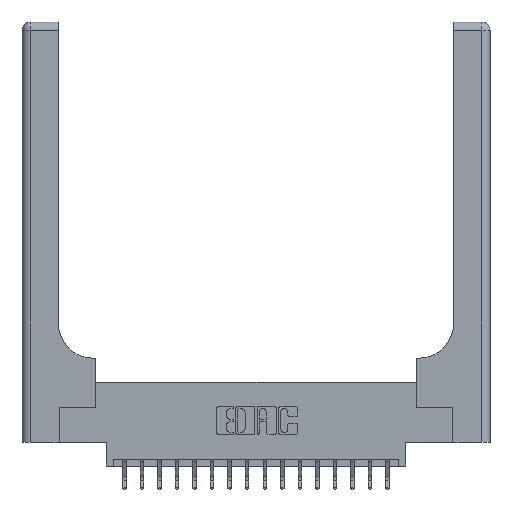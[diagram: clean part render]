
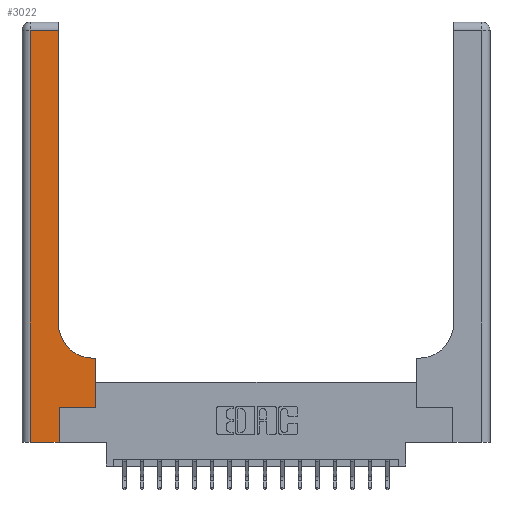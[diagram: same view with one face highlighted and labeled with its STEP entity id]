
A CAD part, top view. The second image highlights one B-rep face of the part: STEP entity #3022.
In plain terms, the highlighted planar face has unit normal (0, 0, 1).
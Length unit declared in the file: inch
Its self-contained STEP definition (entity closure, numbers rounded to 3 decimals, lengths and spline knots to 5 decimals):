
#124 = VECTOR ( 'NONE', #13256, 39.37008 ) ;
#356 = AXIS2_PLACEMENT_3D ( 'NONE', #17560, #8600, #19042 ) ;
#387 = CIRCLE ( 'NONE', #356, 0.25 ) ;
#470 = CARTESIAN_POINT ( 'NONE',  ( 0.26, 2.94, 0.37 ) ) ;
#877 = DIRECTION ( 'NONE',  ( -1., 0., 0. ) ) ;
#941 = EDGE_LOOP ( 'NONE', ( #1233, #9924, #9401, #5810, #12615, #2392, #7498, #4739, #6015 ) ) ;
#948 = CARTESIAN_POINT ( 'NONE',  ( 0.265, 0.25, 0.37 ) ) ;
#1233 = ORIENTED_EDGE ( 'NONE', *, *, #8392, .T. ) ;
#1277 = VERTEX_POINT ( 'NONE', #470 ) ;
#1397 = CARTESIAN_POINT ( 'NONE',  ( 0.06, 2.94, 0.37 ) ) ;
#1507 = CARTESIAN_POINT ( 'NONE',  ( 0.26, 0.85, 0.37 ) ) ;
#1747 = EDGE_CURVE ( 'NONE', #13951, #7354, #18342, .T. ) ;
#1796 = DIRECTION ( 'NONE',  ( 0., 1., 0. ) ) ;
#2098 = VERTEX_POINT ( 'NONE', #19387 ) ;
#2392 = ORIENTED_EDGE ( 'NONE', *, *, #11087, .T. ) ;
#2515 = CARTESIAN_POINT ( 'NONE',  ( 0.26, 0.6, 0.37 ) ) ;
#2745 = CARTESIAN_POINT ( 'NONE',  ( 0.06, 3., 0.37 ) ) ;
#3022 = ADVANCED_FACE ( 'NONE', ( #7053 ), #17415, .F. ) ;
#3240 = VERTEX_POINT ( 'NONE', #1397 ) ;
#3827 = LINE ( 'NONE', #2515, #18836 ) ;
#4114 = VECTOR ( 'NONE', #15551, 39.37008 ) ;
#4638 = CARTESIAN_POINT ( 'NONE',  ( 0.51, 0.6, 0.37 ) ) ;
#4739 = ORIENTED_EDGE ( 'NONE', *, *, #7251, .T. ) ;
#5372 = EDGE_CURVE ( 'NONE', #11642, #6927, #10032, .T. ) ;
#5810 = ORIENTED_EDGE ( 'NONE', *, *, #16534, .T. ) ;
#6015 = ORIENTED_EDGE ( 'NONE', *, *, #15964, .T. ) ;
#6381 = VECTOR ( 'NONE', #1796, 39.37008 ) ;
#6927 = VERTEX_POINT ( 'NONE', #9258 ) ;
#7053 = FACE_OUTER_BOUND ( 'NONE', #941, .T. ) ;
#7251 = EDGE_CURVE ( 'NONE', #6927, #12770, #3827, .T. ) ;
#7315 = LINE ( 'NONE', #948, #17858 ) ;
#7354 = VERTEX_POINT ( 'NONE', #17809 ) ;
#7498 = ORIENTED_EDGE ( 'NONE', *, *, #5372, .T. ) ;
#8170 = CARTESIAN_POINT ( 'NONE',  ( 0.265, 0., 0.37 ) ) ;
#8392 = EDGE_CURVE ( 'NONE', #18990, #1277, #12119, .T. ) ;
#8447 = CARTESIAN_POINT ( 'NONE',  ( 0., 3., 0.37 ) ) ;
#8600 = DIRECTION ( 'NONE',  ( 0., 0., -1. ) ) ;
#9258 = CARTESIAN_POINT ( 'NONE',  ( 0.528, 0.6, 0.37 ) ) ;
#9401 = ORIENTED_EDGE ( 'NONE', *, *, #11819, .T. ) ;
#9924 = ORIENTED_EDGE ( 'NONE', *, *, #13199, .T. ) ;
#9960 = DIRECTION ( 'NONE',  ( 0., 0., -1. ) ) ;
#10032 = LINE ( 'NONE', #14235, #10484 ) ;
#10038 = DIRECTION ( 'NONE',  ( -1., 0., 0. ) ) ;
#10258 = DIRECTION ( 'NONE',  ( 0., -1., 0. ) ) ;
#10350 = VECTOR ( 'NONE', #14552, 39.37008 ) ;
#10484 = VECTOR ( 'NONE', #11203, 39.37008 ) ;
#11041 = CARTESIAN_POINT ( 'NONE',  ( 0.265, 0., 0.37 ) ) ;
#11087 = EDGE_CURVE ( 'NONE', #7354, #11642, #7315, .T. ) ;
#11203 = DIRECTION ( 'NONE',  ( 0., 1., 0. ) ) ;
#11292 = LINE ( 'NONE', #13043, #10350 ) ;
#11642 = VERTEX_POINT ( 'NONE', #15629 ) ;
#11819 = EDGE_CURVE ( 'NONE', #3240, #2098, #12267, .T. ) ;
#12119 = LINE ( 'NONE', #14072, #4114 ) ;
#12267 = LINE ( 'NONE', #2745, #18794 ) ;
#12615 = ORIENTED_EDGE ( 'NONE', *, *, #1747, .T. ) ;
#12770 = VERTEX_POINT ( 'NONE', #4638 ) ;
#13043 = CARTESIAN_POINT ( 'NONE',  ( 0., 0., 0.37 ) ) ;
#13199 = EDGE_CURVE ( 'NONE', #1277, #3240, #15708, .T. ) ;
#13256 = DIRECTION ( 'NONE',  ( -1., 0., 0. ) ) ;
#13951 = VERTEX_POINT ( 'NONE', #11041 ) ;
#14072 = CARTESIAN_POINT ( 'NONE',  ( 0.26, 3., 0.37 ) ) ;
#14235 = CARTESIAN_POINT ( 'NONE',  ( 0.528, 0.25, 0.37 ) ) ;
#14552 = DIRECTION ( 'NONE',  ( 1., 0., 0. ) ) ;
#15551 = DIRECTION ( 'NONE',  ( 0., 1., 0. ) ) ;
#15629 = CARTESIAN_POINT ( 'NONE',  ( 0.528, 0.25, 0.37 ) ) ;
#15708 = LINE ( 'NONE', #19497, #124 ) ;
#15964 = EDGE_CURVE ( 'NONE', #12770, #18990, #387, .T. ) ;
#16049 = DIRECTION ( 'NONE',  ( 1., 0., 0. ) ) ;
#16534 = EDGE_CURVE ( 'NONE', #2098, #13951, #11292, .T. ) ;
#17415 = PLANE ( 'NONE',  #17582 ) ;
#17560 = CARTESIAN_POINT ( 'NONE',  ( 0.51, 0.85, 0.37 ) ) ;
#17582 = AXIS2_PLACEMENT_3D ( 'NONE', #8447, #9960, #877 ) ;
#17809 = CARTESIAN_POINT ( 'NONE',  ( 0.265, 0.25, 0.37 ) ) ;
#17858 = VECTOR ( 'NONE', #16049, 39.37008 ) ;
#18342 = LINE ( 'NONE', #8170, #6381 ) ;
#18794 = VECTOR ( 'NONE', #10258, 39.37008 ) ;
#18836 = VECTOR ( 'NONE', #10038, 39.37008 ) ;
#18990 = VERTEX_POINT ( 'NONE', #1507 ) ;
#19042 = DIRECTION ( 'NONE',  ( 1., 0., 0. ) ) ;
#19387 = CARTESIAN_POINT ( 'NONE',  ( 0.06, 0., 0.37 ) ) ;
#19497 = CARTESIAN_POINT ( 'NONE',  ( 0., 2.94, 0.37 ) ) ;
